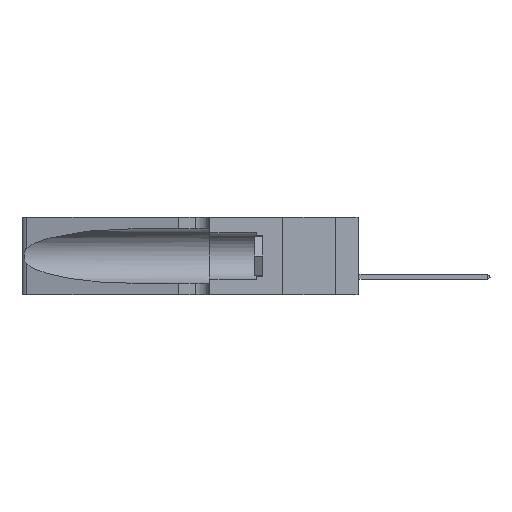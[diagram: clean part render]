
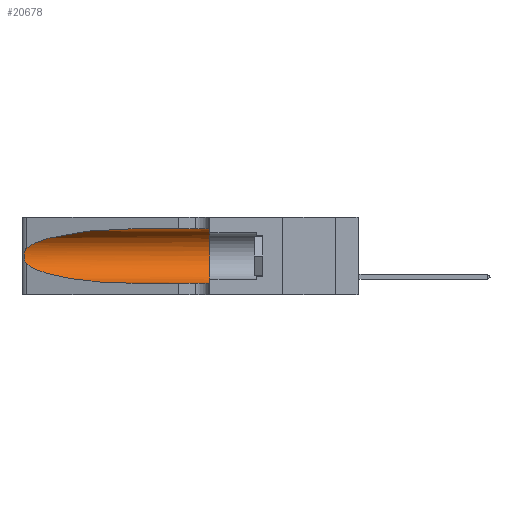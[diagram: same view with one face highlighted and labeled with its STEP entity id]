
A CAD part, left-side view. The second image highlights one B-rep face of the part: STEP entity #20678.
In plain terms, the highlighted cylindrical face has radius 3.308 mm (diameter 6.617 mm), a partial arc.
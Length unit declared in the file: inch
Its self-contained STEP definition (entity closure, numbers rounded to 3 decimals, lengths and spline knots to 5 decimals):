
#515 = CARTESIAN_POINT ( 'NONE',  ( 0.25856, 1.23593, 0.16098 ) ) ;
#601 = CARTESIAN_POINT ( 'NONE',  ( 0.26075, 1.23896, 0.178 ) ) ;
#775 = EDGE_CURVE ( 'NONE', #3610, #19232, #11371, .T. ) ;
#1266 = FACE_OUTER_BOUND ( 'NONE', #7946, .T. ) ;
#1396 = ORIENTED_EDGE ( 'NONE', *, *, #7749, .F. ) ;
#1868 = VERTEX_POINT ( 'NONE', #12120 ) ;
#1898 = VERTEX_POINT ( 'NONE', #17781 ) ;
#2239 = CARTESIAN_POINT ( 'NONE',  ( 0.2373, 1.15595, 0.08982 ) ) ;
#2759 = DIRECTION ( 'NONE',  ( 0., 0., -1. ) ) ;
#2931 = VECTOR ( 'NONE', #13903, 39.37008 ) ;
#3610 = VERTEX_POINT ( 'NONE', #10525 ) ;
#3819 = CARTESIAN_POINT ( 'NONE',  ( 0.1305, 1.61858, 0.185 ) ) ;
#3996 = EDGE_CURVE ( 'NONE', #19592, #1898, #22572, .T. ) ;
#4435 = CARTESIAN_POINT ( 'NONE',  ( 0.26017, 1.23833, 0.17102 ) ) ;
#5049 = AXIS2_PLACEMENT_3D ( 'NONE', #24521, #5665, #7243 ) ;
#5665 = DIRECTION ( 'NONE',  ( 0., 1., 0. ) ) ;
#5962 = VECTOR ( 'NONE', #24550, 39.37008 ) ;
#6119 = CARTESIAN_POINT ( 'NONE',  ( 0.25487, 1.22718, 0.14631 ) ) ;
#6202 = CARTESIAN_POINT ( 'NONE',  ( 0.18966, 0.96281, 0.05475 ) ) ;
#6307 = CARTESIAN_POINT ( 'NONE',  ( 0.1305, 0.72297, 0.31525 ) ) ;
#6393 = CARTESIAN_POINT ( 'NONE',  ( 0.25789, 1.23486, 0.15765 ) ) ;
#7243 = DIRECTION ( 'NONE',  ( 0., 0., 1. ) ) ;
#7749 = EDGE_CURVE ( 'NONE', #19165, #1868, #11430, .T. ) ;
#7946 = EDGE_LOOP ( 'NONE', ( #13418, #15678, #16295, #16472, #1396, #24398 ) ) ;
#8073 = CARTESIAN_POINT ( 'NONE',  ( 0.2373, 1.15595, 0.28018 ) ) ;
#8230 = CARTESIAN_POINT ( 'NONE',  ( 0.25487, 1.22718, 0.22369 ) ) ;
#8318 = CARTESIAN_POINT ( 'NONE',  ( 0.25487, 1.22718, 0.14631 ) ) ;
#9982 = CARTESIAN_POINT ( 'NONE',  ( 0.26075, 1.23896, 0.19203 ) ) ;
#10000 = CARTESIAN_POINT ( 'NONE',  ( 0.1305, 1.61858, 0.31525 ) ) ;
#10525 = CARTESIAN_POINT ( 'NONE',  ( 0.25487, 1.22718, 0.14631 ) ) ;
#11371 =( BOUNDED_CURVE ( )  B_SPLINE_CURVE ( 3, ( #6119, #2239, #6202, #19549 ),
 .UNSPECIFIED., .F., .F. ) 
 B_SPLINE_CURVE_WITH_KNOTS ( ( 4, 4 ),
 ( 3.44316, 4.71239 ),
 .UNSPECIFIED. ) 
 CURVE ( )  GEOMETRIC_REPRESENTATION_ITEM ( )  RATIONAL_B_SPLINE_CURVE ( ( 1., 0.87, 0.87, 1. ) ) 
 REPRESENTATION_ITEM ( '' )  );
#11430 = CIRCLE ( 'NONE', #5049, 0.13025 ) ;
#11894 = CARTESIAN_POINT ( 'NONE',  ( 0.25639, 1.23186, 0.15144 ) ) ;
#11973 = CARTESIAN_POINT ( 'NONE',  ( 0.25854, 1.2359, 0.20912 ) ) ;
#12120 = CARTESIAN_POINT ( 'NONE',  ( 0.1305, 0.35, 0.05475 ) ) ;
#12848 = CARTESIAN_POINT ( 'NONE',  ( 0.1305, 1.61858, 0.05475 ) ) ;
#13059 = LINE ( 'NONE', #10000, #2931 ) ;
#13414 = LINE ( 'NONE', #12848, #5962 ) ;
#13418 = ORIENTED_EDGE ( 'NONE', *, *, #3996, .T. ) ;
#13808 = CARTESIAN_POINT ( 'NONE',  ( 0.25787, 1.23484, 0.2124 ) ) ;
#13903 = DIRECTION ( 'NONE',  ( 0., -1., 0. ) ) ;
#13918 = CARTESIAN_POINT ( 'NONE',  ( 0.1305, 0.72297, 0.31525 ) ) ;
#15639 = EDGE_CURVE ( 'NONE', #19232, #1868, #13414, .T. ) ;
#15678 = ORIENTED_EDGE ( 'NONE', *, *, #17145, .T. ) ;
#16295 = ORIENTED_EDGE ( 'NONE', *, *, #775, .T. ) ;
#16472 = ORIENTED_EDGE ( 'NONE', *, *, #15639, .T. ) ;
#16998 = AXIS2_PLACEMENT_3D ( 'NONE', #3819, #21782, #2759 ) ;
#17145 = EDGE_CURVE ( 'NONE', #1898, #3610, #23321, .T. ) ;
#17710 = CARTESIAN_POINT ( 'NONE',  ( 0.18966, 0.96281, 0.31525 ) ) ;
#17781 = CARTESIAN_POINT ( 'NONE',  ( 0.25487, 1.22718, 0.22369 ) ) ;
#17806 = CARTESIAN_POINT ( 'NONE',  ( 0.25639, 1.23184, 0.21858 ) ) ;
#19165 = VERTEX_POINT ( 'NONE', #20899 ) ;
#19232 = VERTEX_POINT ( 'NONE', #23213 ) ;
#19549 = CARTESIAN_POINT ( 'NONE',  ( 0.1305, 0.72297, 0.05475 ) ) ;
#19592 = VERTEX_POINT ( 'NONE', #13918 ) ;
#19747 = CARTESIAN_POINT ( 'NONE',  ( 0.25555, 1.22994, 0.2215 ) ) ;
#19827 = CARTESIAN_POINT ( 'NONE',  ( 0.25555, 1.22993, 0.14849 ) ) ;
#20049 = CYLINDRICAL_SURFACE ( 'NONE', #16998, 0.13025 ) ;
#20678 = ADVANCED_FACE ( 'NONE', ( #1266 ), #20049, .F. ) ;
#20899 = CARTESIAN_POINT ( 'NONE',  ( 0.1305, 0.35, 0.31525 ) ) ;
#21450 = CARTESIAN_POINT ( 'NONE',  ( 0.26018, 1.23835, 0.19895 ) ) ;
#21768 = CARTESIAN_POINT ( 'NONE',  ( 0.25487, 1.22718, 0.22369 ) ) ;
#21782 = DIRECTION ( 'NONE',  ( 0., -1., 0. ) ) ;
#22572 =( BOUNDED_CURVE ( )  B_SPLINE_CURVE ( 3, ( #6307, #17710, #8073, #21768 ),
 .UNSPECIFIED., .F., .F. ) 
 B_SPLINE_CURVE_WITH_KNOTS ( ( 4, 4 ),
 ( 1.5708, 2.84003 ),
 .UNSPECIFIED. ) 
 CURVE ( )  GEOMETRIC_REPRESENTATION_ITEM ( )  RATIONAL_B_SPLINE_CURVE ( ( 1., 0.87, 0.87, 1. ) ) 
 REPRESENTATION_ITEM ( '' )  );
#23213 = CARTESIAN_POINT ( 'NONE',  ( 0.1305, 0.72297, 0.05475 ) ) ;
#23321 = B_SPLINE_CURVE_WITH_KNOTS ( 'NONE', 3,
 ( #8230, #19747, #17806, #13808, #11973, #21450, #9982, #601, #4435, #515, #6393, #11894, #19827, #8318 ),
 .UNSPECIFIED., .F., .F.,
 ( 4, 2, 2, 2, 2, 2, 4 ),
 ( 0., 0.00027, 0.00053, 0.00107, 0.0016, 0.00187, 0.00214 ),
 .UNSPECIFIED. ) ;
#23685 = EDGE_CURVE ( 'NONE', #19592, #19165, #13059, .T. ) ;
#24398 = ORIENTED_EDGE ( 'NONE', *, *, #23685, .F. ) ;
#24521 = CARTESIAN_POINT ( 'NONE',  ( 0.1305, 0.35, 0.185 ) ) ;
#24550 = DIRECTION ( 'NONE',  ( 0., -1., 0. ) ) ;
